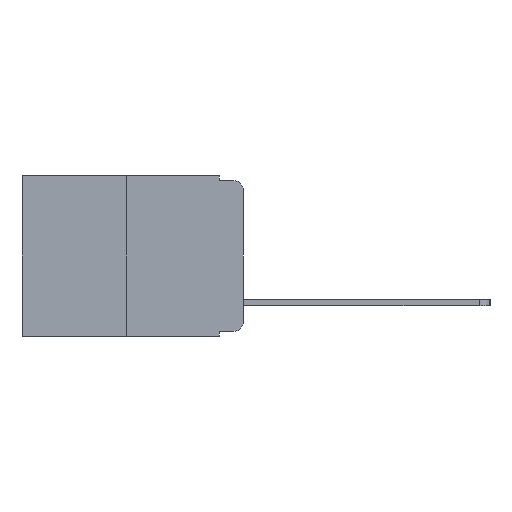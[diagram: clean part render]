
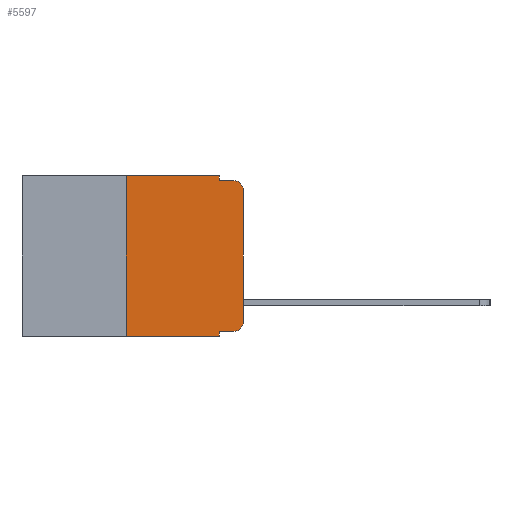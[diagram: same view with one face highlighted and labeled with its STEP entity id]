
A CAD part, left-side view. The second image highlights one B-rep face of the part: STEP entity #5597.
In plain terms, the highlighted planar face has unit normal (-1, 0, 0).
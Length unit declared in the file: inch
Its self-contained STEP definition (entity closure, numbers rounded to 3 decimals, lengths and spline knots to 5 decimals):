
#25 = CARTESIAN_POINT ( 'NONE',  ( 0., 0.473, 0. ) ) ;
#30 = EDGE_CURVE ( 'NONE', #736, #4039, #4151, .T. ) ;
#53 = DIRECTION ( 'NONE',  ( -1., 0., 0. ) ) ;
#140 = VERTEX_POINT ( 'NONE', #973 ) ;
#384 = PLANE ( 'NONE',  #10112 ) ;
#430 = LINE ( 'NONE', #2576, #7454 ) ;
#433 = CARTESIAN_POINT ( 'NONE',  ( 0., 0.25, 0. ) ) ;
#660 = EDGE_CURVE ( 'NONE', #1549, #736, #9961, .T. ) ;
#735 = CARTESIAN_POINT ( 'NONE',  ( 0., 0.25, -0.343 ) ) ;
#736 = VERTEX_POINT ( 'NONE', #3221 ) ;
#759 = CARTESIAN_POINT ( 'NONE',  ( 0., 0.051, -0.333 ) ) ;
#801 = VERTEX_POINT ( 'NONE', #6726 ) ;
#889 = VERTEX_POINT ( 'NONE', #433 ) ;
#902 = AXIS2_PLACEMENT_3D ( 'NONE', #7240, #1836, #8055 ) ;
#909 = CARTESIAN_POINT ( 'NONE',  ( 0., 0.051, 0. ) ) ;
#973 = CARTESIAN_POINT ( 'NONE',  ( 0., 0.051, -0.01 ) ) ;
#1030 = DIRECTION ( 'NONE',  ( 0., 0., 1. ) ) ;
#1198 = VECTOR ( 'NONE', #6523, 39.37008 ) ;
#1270 = ORIENTED_EDGE ( 'NONE', *, *, #3857, .F. ) ;
#1372 = DIRECTION ( 'NONE',  ( 1., 0., 0. ) ) ;
#1444 = DIRECTION ( 'NONE',  ( 0., -1., 0. ) ) ;
#1512 = VECTOR ( 'NONE', #2046, 39.37008 ) ;
#1549 = VERTEX_POINT ( 'NONE', #9618 ) ;
#1598 = ORIENTED_EDGE ( 'NONE', *, *, #2641, .F. ) ;
#1627 = LINE ( 'NONE', #10522, #10572 ) ;
#1836 = DIRECTION ( 'NONE',  ( -1., 0., 0. ) ) ;
#2011 = EDGE_CURVE ( 'NONE', #1549, #4925, #3538, .T. ) ;
#2046 = DIRECTION ( 'NONE',  ( 0., 0., -1. ) ) ;
#2440 = AXIS2_PLACEMENT_3D ( 'NONE', #10611, #53, #6552 ) ;
#2564 = FACE_OUTER_BOUND ( 'NONE', #4872, .T. ) ;
#2576 = CARTESIAN_POINT ( 'NONE',  ( 0., 0.051, -0.01 ) ) ;
#2602 = VERTEX_POINT ( 'NONE', #4210 ) ;
#2641 = EDGE_CURVE ( 'NONE', #3030, #889, #11269, .T. ) ;
#3030 = VERTEX_POINT ( 'NONE', #735 ) ;
#3109 = CARTESIAN_POINT ( 'NONE',  ( 0., 0.051, 0. ) ) ;
#3221 = CARTESIAN_POINT ( 'NONE',  ( 0., 0.02, -0.333 ) ) ;
#3538 = LINE ( 'NONE', #3109, #5683 ) ;
#3696 = DIRECTION ( 'NONE',  ( 0., 0., 1. ) ) ;
#3797 = ORIENTED_EDGE ( 'NONE', *, *, #3877, .F. ) ;
#3857 = EDGE_CURVE ( 'NONE', #5192, #140, #8366, .T. ) ;
#3877 = EDGE_CURVE ( 'NONE', #889, #5192, #9976, .T. ) ;
#4033 = DIRECTION ( 'NONE',  ( 0., 0., -1. ) ) ;
#4039 = VERTEX_POINT ( 'NONE', #10376 ) ;
#4151 = CIRCLE ( 'NONE', #2440, 0.02 ) ;
#4210 = CARTESIAN_POINT ( 'NONE',  ( 0., 0., -0.03 ) ) ;
#4490 = EDGE_CURVE ( 'NONE', #140, #801, #430, .T. ) ;
#4758 = CIRCLE ( 'NONE', #902, 0.02 ) ;
#4872 = EDGE_LOOP ( 'NONE', ( #5400, #5662, #7900, #1270, #3797, #1598, #6469, #6740, #8689, #8936 ) ) ;
#4925 = VERTEX_POINT ( 'NONE', #5302 ) ;
#5118 = EDGE_CURVE ( 'NONE', #2602, #801, #4758, .T. ) ;
#5192 = VERTEX_POINT ( 'NONE', #909 ) ;
#5302 = CARTESIAN_POINT ( 'NONE',  ( 0., 0.051, -0.343 ) ) ;
#5400 = ORIENTED_EDGE ( 'NONE', *, *, #5702, .T. ) ;
#5575 = VECTOR ( 'NONE', #1444, 39.37008 ) ;
#5596 = DIRECTION ( 'NONE',  ( 0., -1., 0. ) ) ;
#5597 = ADVANCED_FACE ( 'NONE', ( #2564 ), #384, .F. ) ;
#5662 = ORIENTED_EDGE ( 'NONE', *, *, #5118, .T. ) ;
#5683 = VECTOR ( 'NONE', #4033, 39.37008 ) ;
#5699 = CARTESIAN_POINT ( 'NONE',  ( 0., 0., 0. ) ) ;
#5702 = EDGE_CURVE ( 'NONE', #4039, #2602, #10588, .T. ) ;
#6060 = CARTESIAN_POINT ( 'NONE',  ( 0., 0.473, 0. ) ) ;
#6469 = ORIENTED_EDGE ( 'NONE', *, *, #10456, .T. ) ;
#6523 = DIRECTION ( 'NONE',  ( 0., -1., 0. ) ) ;
#6552 = DIRECTION ( 'NONE',  ( 0., 0., -1. ) ) ;
#6726 = CARTESIAN_POINT ( 'NONE',  ( 0., 0.02, -0.01 ) ) ;
#6740 = ORIENTED_EDGE ( 'NONE', *, *, #2011, .F. ) ;
#7240 = CARTESIAN_POINT ( 'NONE',  ( 0., 0.02, -0.03 ) ) ;
#7454 = VECTOR ( 'NONE', #8700, 39.37008 ) ;
#7688 = DIRECTION ( 'NONE',  ( 0., 0., -1. ) ) ;
#7900 = ORIENTED_EDGE ( 'NONE', *, *, #4490, .F. ) ;
#8055 = DIRECTION ( 'NONE',  ( 0., 0., -1. ) ) ;
#8077 = CARTESIAN_POINT ( 'NONE',  ( 0., 0.25, 0. ) ) ;
#8198 = VECTOR ( 'NONE', #1030, 39.37008 ) ;
#8366 = LINE ( 'NONE', #10621, #1512 ) ;
#8689 = ORIENTED_EDGE ( 'NONE', *, *, #660, .T. ) ;
#8700 = DIRECTION ( 'NONE',  ( 0., -1., 0. ) ) ;
#8936 = ORIENTED_EDGE ( 'NONE', *, *, #30, .T. ) ;
#9618 = CARTESIAN_POINT ( 'NONE',  ( 0., 0.051, -0.333 ) ) ;
#9961 = LINE ( 'NONE', #759, #5575 ) ;
#9976 = LINE ( 'NONE', #25, #1198 ) ;
#10112 = AXIS2_PLACEMENT_3D ( 'NONE', #6060, #1372, #7688 ) ;
#10376 = CARTESIAN_POINT ( 'NONE',  ( 0., 0., -0.313 ) ) ;
#10456 = EDGE_CURVE ( 'NONE', #3030, #4925, #1627, .T. ) ;
#10522 = CARTESIAN_POINT ( 'NONE',  ( 0., 0.473, -0.343 ) ) ;
#10572 = VECTOR ( 'NONE', #5596, 39.37008 ) ;
#10588 = LINE ( 'NONE', #5699, #8198 ) ;
#10611 = CARTESIAN_POINT ( 'NONE',  ( 0., 0.02, -0.313 ) ) ;
#10621 = CARTESIAN_POINT ( 'NONE',  ( 0., 0.051, 0. ) ) ;
#11014 = VECTOR ( 'NONE', #3696, 39.37008 ) ;
#11269 = LINE ( 'NONE', #8077, #11014 ) ;
